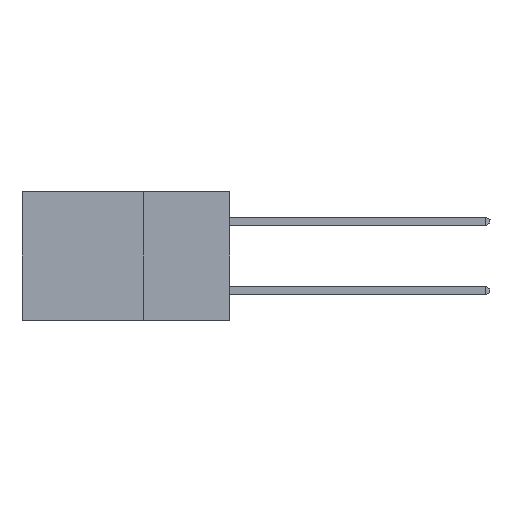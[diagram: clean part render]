
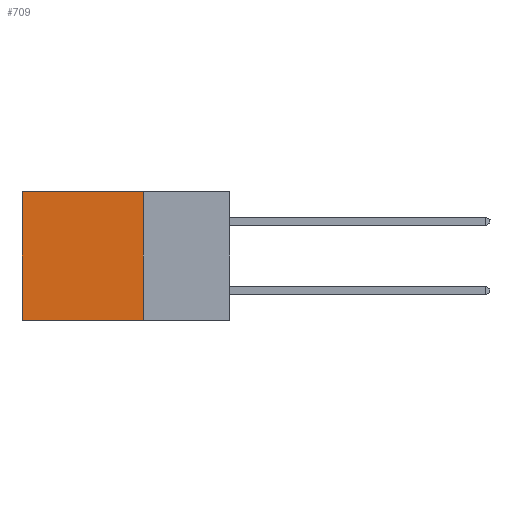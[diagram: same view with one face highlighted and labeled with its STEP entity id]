
A CAD part, left-side view. The second image highlights one B-rep face of the part: STEP entity #709.
In plain terms, the highlighted planar face has unit normal (-1, 0, 0).
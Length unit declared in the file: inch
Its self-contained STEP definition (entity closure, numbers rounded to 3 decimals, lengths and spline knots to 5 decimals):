
#95 = CARTESIAN_POINT ( 'NONE',  ( 0.298, 0.25, 0. ) ) ;
#159 = VECTOR ( 'NONE', #17147, 39.37008 ) ;
#580 = CARTESIAN_POINT ( 'NONE',  ( 0.298, 0.6, -0.37 ) ) ;
#701 = EDGE_CURVE ( 'NONE', #16298, #2694, #26585, .T. ) ;
#709 = ADVANCED_FACE ( 'NONE', ( #14762 ), #26061, .F. ) ;
#740 = LINE ( 'NONE', #95, #21954 ) ;
#842 = ORIENTED_EDGE ( 'NONE', *, *, #701, .F. ) ;
#2569 = ORIENTED_EDGE ( 'NONE', *, *, #8014, .F. ) ;
#2694 = VERTEX_POINT ( 'NONE', #580 ) ;
#3344 = ORIENTED_EDGE ( 'NONE', *, *, #9756, .T. ) ;
#3757 = EDGE_LOOP ( 'NONE', ( #19733, #842, #2569, #3344 ) ) ;
#3798 = VERTEX_POINT ( 'NONE', #23335 ) ;
#4012 = CARTESIAN_POINT ( 'NONE',  ( 0.298, 0.6, 0. ) ) ;
#4037 = CARTESIAN_POINT ( 'NONE',  ( 0.298, 0.25, -0.37 ) ) ;
#4265 = EDGE_CURVE ( 'NONE', #24746, #2694, #6382, .T. ) ;
#5882 = LINE ( 'NONE', #6656, #159 ) ;
#6382 = LINE ( 'NONE', #4012, #15583 ) ;
#6656 = CARTESIAN_POINT ( 'NONE',  ( 0.298, 0.25, 0. ) ) ;
#8014 = EDGE_CURVE ( 'NONE', #3798, #16298, #5882, .T. ) ;
#9756 = EDGE_CURVE ( 'NONE', #3798, #24746, #740, .T. ) ;
#10876 = CARTESIAN_POINT ( 'NONE',  ( 0.298, 0.25, 0. ) ) ;
#14424 = DIRECTION ( 'NONE',  ( 0., 0., -1. ) ) ;
#14762 = FACE_OUTER_BOUND ( 'NONE', #3757, .T. ) ;
#15583 = VECTOR ( 'NONE', #14424, 39.37008 ) ;
#16298 = VERTEX_POINT ( 'NONE', #4037 ) ;
#17147 = DIRECTION ( 'NONE',  ( 0., 0., -1. ) ) ;
#19083 = DIRECTION ( 'NONE',  ( 0., 1., 0. ) ) ;
#19289 = CARTESIAN_POINT ( 'NONE',  ( 0.298, 0.25, -0.37 ) ) ;
#19733 = ORIENTED_EDGE ( 'NONE', *, *, #4265, .T. ) ;
#20412 = VECTOR ( 'NONE', #20932, 39.37008 ) ;
#20932 = DIRECTION ( 'NONE',  ( 0., 1., 0. ) ) ;
#21854 = CARTESIAN_POINT ( 'NONE',  ( 0.298, 0.6, 0. ) ) ;
#21889 = DIRECTION ( 'NONE',  ( 0., 0., -1. ) ) ;
#21954 = VECTOR ( 'NONE', #19083, 39.37008 ) ;
#22730 = AXIS2_PLACEMENT_3D ( 'NONE', #10876, #26148, #21889 ) ;
#23335 = CARTESIAN_POINT ( 'NONE',  ( 0.298, 0.25, 0. ) ) ;
#24746 = VERTEX_POINT ( 'NONE', #21854 ) ;
#26061 = PLANE ( 'NONE',  #22730 ) ;
#26148 = DIRECTION ( 'NONE',  ( 1., 0., 0. ) ) ;
#26585 = LINE ( 'NONE', #19289, #20412 ) ;
